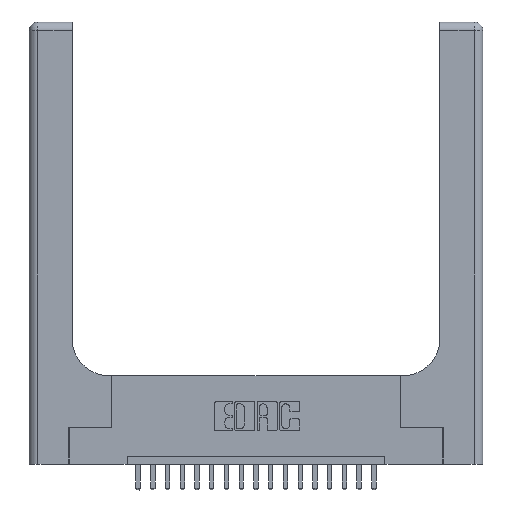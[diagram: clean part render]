
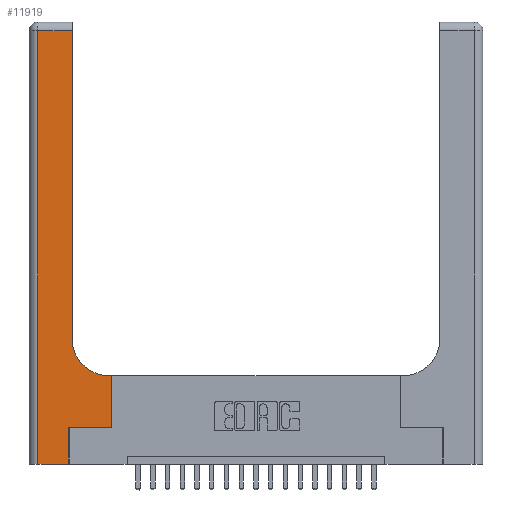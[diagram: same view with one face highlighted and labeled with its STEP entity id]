
A CAD part, top view. The second image highlights one B-rep face of the part: STEP entity #11919.
In plain terms, the highlighted planar face has unit normal (0, 0, 1).
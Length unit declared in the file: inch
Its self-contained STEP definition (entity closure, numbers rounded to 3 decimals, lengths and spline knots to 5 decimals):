
#36 = CARTESIAN_POINT ( 'NONE',  ( 0., 0., 0.37 ) ) ;
#356 = CARTESIAN_POINT ( 'NONE',  ( 0.269, 0.25, 0.37 ) ) ;
#712 = VECTOR ( 'NONE', #16862, 39.37008 ) ;
#1061 = ORIENTED_EDGE ( 'NONE', *, *, #14497, .T. ) ;
#1304 = CARTESIAN_POINT ( 'NONE',  ( 0.06, 0., 0.37 ) ) ;
#1846 = VERTEX_POINT ( 'NONE', #14236 ) ;
#1854 = VECTOR ( 'NONE', #20685, 39.37008 ) ;
#1882 = DIRECTION ( 'NONE',  ( 0., 1., 0. ) ) ;
#2017 = VERTEX_POINT ( 'NONE', #9595 ) ;
#2287 = LINE ( 'NONE', #9851, #15296 ) ;
#2374 = EDGE_CURVE ( 'NONE', #7724, #11018, #14310, .T. ) ;
#2546 = PLANE ( 'NONE',  #17590 ) ;
#2653 = EDGE_CURVE ( 'NONE', #8692, #7724, #4439, .T. ) ;
#2661 = DIRECTION ( 'NONE',  ( 0., 0., -1. ) ) ;
#3032 = LINE ( 'NONE', #13060, #18854 ) ;
#3118 = EDGE_CURVE ( 'NONE', #1846, #15384, #15074, .T. ) ;
#3214 = DIRECTION ( 'NONE',  ( -1., 0., 0. ) ) ;
#3547 = DIRECTION ( 'NONE',  ( 1., 0., 0. ) ) ;
#4126 = EDGE_CURVE ( 'NONE', #8157, #1846, #20182, .T. ) ;
#4439 = LINE ( 'NONE', #8101, #14571 ) ;
#4511 = CARTESIAN_POINT ( 'NONE',  ( 0.269, 0.25, 0.37 ) ) ;
#4924 = DIRECTION ( 'NONE',  ( -1., 0., 0. ) ) ;
#5029 = ORIENTED_EDGE ( 'NONE', *, *, #2653, .T. ) ;
#5692 = CARTESIAN_POINT ( 'NONE',  ( 0., 3., 0.37 ) ) ;
#6717 = CARTESIAN_POINT ( 'NONE',  ( 0.2915, 2.94, 0.37 ) ) ;
#6839 = EDGE_CURVE ( 'NONE', #2017, #8692, #10442, .T. ) ;
#6951 = ORIENTED_EDGE ( 'NONE', *, *, #13806, .T. ) ;
#7724 = VERTEX_POINT ( 'NONE', #19390 ) ;
#7916 = ORIENTED_EDGE ( 'NONE', *, *, #21120, .T. ) ;
#8101 = CARTESIAN_POINT ( 'NONE',  ( 0., 2.94, 0.37 ) ) ;
#8157 = VERTEX_POINT ( 'NONE', #4511 ) ;
#8692 = VERTEX_POINT ( 'NONE', #6717 ) ;
#9362 = VERTEX_POINT ( 'NONE', #20643 ) ;
#9473 = CARTESIAN_POINT ( 'NONE',  ( 0.5415, 0.85, 0.37 ) ) ;
#9595 = CARTESIAN_POINT ( 'NONE',  ( 0.2915, 0.85, 0.37 ) ) ;
#9627 = ORIENTED_EDGE ( 'NONE', *, *, #9853, .T. ) ;
#9851 = CARTESIAN_POINT ( 'NONE',  ( 0.2915, 0.6, 0.37 ) ) ;
#9853 = EDGE_CURVE ( 'NONE', #15384, #9362, #2287, .T. ) ;
#10060 = DIRECTION ( 'NONE',  ( 0., 1., 0. ) ) ;
#10070 = FACE_OUTER_BOUND ( 'NONE', #15101, .T. ) ;
#10292 = CARTESIAN_POINT ( 'NONE',  ( 0.269, 0., 0.37 ) ) ;
#10442 = LINE ( 'NONE', #20000, #19769 ) ;
#10522 = CIRCLE ( 'NONE', #18880, 0.25 ) ;
#10691 = DIRECTION ( 'NONE',  ( -1., 0., 0. ) ) ;
#10763 = DIRECTION ( 'NONE',  ( 0., 0., -1. ) ) ;
#10873 = DIRECTION ( 'NONE',  ( 1., 0., 0. ) ) ;
#11018 = VERTEX_POINT ( 'NONE', #1304 ) ;
#11094 = ORIENTED_EDGE ( 'NONE', *, *, #4126, .T. ) ;
#11919 = ADVANCED_FACE ( 'NONE', ( #10070 ), #2546, .F. ) ;
#13060 = CARTESIAN_POINT ( 'NONE',  ( 0.269, 0., 0.37 ) ) ;
#13287 = ORIENTED_EDGE ( 'NONE', *, *, #3118, .T. ) ;
#13806 = EDGE_CURVE ( 'NONE', #14296, #8157, #3032, .T. ) ;
#14236 = CARTESIAN_POINT ( 'NONE',  ( 0.5585, 0.25, 0.37 ) ) ;
#14296 = VERTEX_POINT ( 'NONE', #10292 ) ;
#14310 = LINE ( 'NONE', #20756, #1854 ) ;
#14497 = EDGE_CURVE ( 'NONE', #9362, #2017, #10522, .T. ) ;
#14571 = VECTOR ( 'NONE', #3214, 39.37008 ) ;
#15074 = LINE ( 'NONE', #21416, #17378 ) ;
#15101 = EDGE_LOOP ( 'NONE', ( #17992, #5029, #18708, #7916, #6951, #11094, #13287, #9627, #1061 ) ) ;
#15296 = VECTOR ( 'NONE', #4924, 39.37008 ) ;
#15384 = VERTEX_POINT ( 'NONE', #18641 ) ;
#16862 = DIRECTION ( 'NONE',  ( 1., 0., 0. ) ) ;
#17378 = VECTOR ( 'NONE', #10060, 39.37008 ) ;
#17590 = AXIS2_PLACEMENT_3D ( 'NONE', #5692, #10763, #10691 ) ;
#17992 = ORIENTED_EDGE ( 'NONE', *, *, #6839, .T. ) ;
#18641 = CARTESIAN_POINT ( 'NONE',  ( 0.5585, 0.6, 0.37 ) ) ;
#18708 = ORIENTED_EDGE ( 'NONE', *, *, #2374, .T. ) ;
#18854 = VECTOR ( 'NONE', #21234, 39.37008 ) ;
#18880 = AXIS2_PLACEMENT_3D ( 'NONE', #9473, #2661, #10873 ) ;
#19390 = CARTESIAN_POINT ( 'NONE',  ( 0.06, 2.94, 0.37 ) ) ;
#19668 = VECTOR ( 'NONE', #3547, 39.37008 ) ;
#19769 = VECTOR ( 'NONE', #1882, 39.37008 ) ;
#20000 = CARTESIAN_POINT ( 'NONE',  ( 0.2915, 3., 0.37 ) ) ;
#20182 = LINE ( 'NONE', #356, #19668 ) ;
#20643 = CARTESIAN_POINT ( 'NONE',  ( 0.5415, 0.6, 0.37 ) ) ;
#20685 = DIRECTION ( 'NONE',  ( 0., -1., 0. ) ) ;
#20756 = CARTESIAN_POINT ( 'NONE',  ( 0.06, 3., 0.37 ) ) ;
#21120 = EDGE_CURVE ( 'NONE', #11018, #14296, #21199, .T. ) ;
#21199 = LINE ( 'NONE', #36, #712 ) ;
#21234 = DIRECTION ( 'NONE',  ( 0., 1., 0. ) ) ;
#21416 = CARTESIAN_POINT ( 'NONE',  ( 0.5585, 0.25, 0.37 ) ) ;
